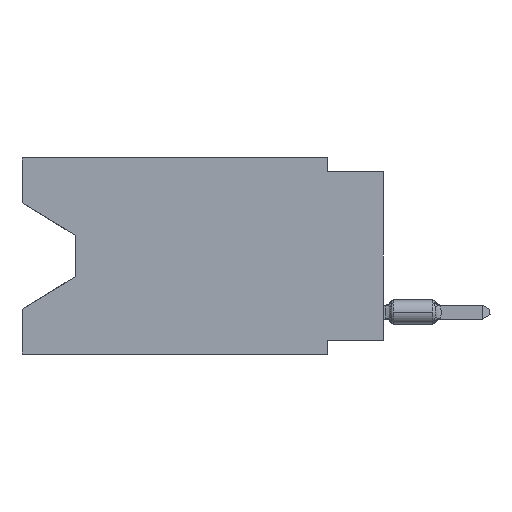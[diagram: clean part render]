
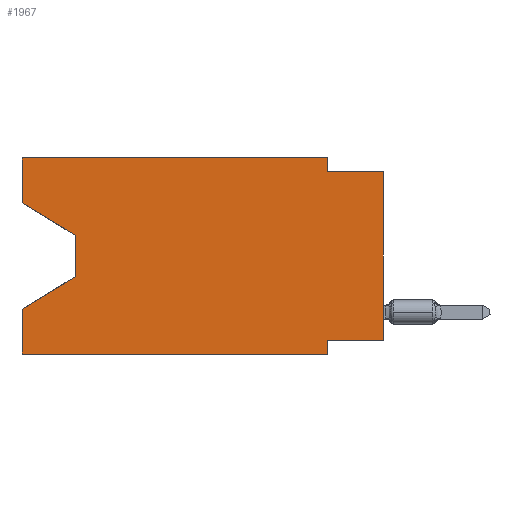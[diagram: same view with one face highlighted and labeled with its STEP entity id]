
A CAD part, left-side view. The second image highlights one B-rep face of the part: STEP entity #1967.
In plain terms, the highlighted planar face has unit normal (-1, 0, 0).
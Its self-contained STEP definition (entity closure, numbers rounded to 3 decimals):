
#152 = EDGE_CURVE ( 'NONE', #29118, #13031, #9220, .T. ) ;
#993 = CARTESIAN_POINT ( 'NONE',  ( 0., 16.383, -8.89 ) ) ;
#1120 = LINE ( 'NONE', #49168, #19352 ) ;
#1580 = CARTESIAN_POINT ( 'NONE',  ( 0., 0., -8.255 ) ) ;
#1967 = ADVANCED_FACE ( 'NONE', ( #51818 ), #21676, .F. ) ;
#2218 = DIRECTION ( 'NONE',  ( 0., -0.855, -0.519 ) ) ;
#2401 = LINE ( 'NONE', #15149, #39441 ) ;
#3089 = ORIENTED_EDGE ( 'NONE', *, *, #32509, .F. ) ;
#3797 = VECTOR ( 'NONE', #8239, 1000. ) ;
#4274 = EDGE_CURVE ( 'NONE', #53425, #5177, #39227, .T. ) ;
#4818 = CARTESIAN_POINT ( 'NONE',  ( 0., 16.383, -2.038 ) ) ;
#5027 = CARTESIAN_POINT ( 'NONE',  ( 0., 13.97, -3.505 ) ) ;
#5177 = VERTEX_POINT ( 'NONE', #44967 ) ;
#6761 = EDGE_CURVE ( 'NONE', #54355, #32090, #35703, .T. ) ;
#7062 = DIRECTION ( 'NONE',  ( 0., 1., 0. ) ) ;
#7073 = CARTESIAN_POINT ( 'NONE',  ( 0., 0., -8.255 ) ) ;
#8239 = DIRECTION ( 'NONE',  ( 0., 0., -1. ) ) ;
#8268 = VECTOR ( 'NONE', #56622, 1000. ) ;
#8330 = EDGE_CURVE ( 'NONE', #24706, #37891, #1120, .T. ) ;
#9220 = LINE ( 'NONE', #35254, #9801 ) ;
#9801 = VECTOR ( 'NONE', #54073, 1000. ) ;
#10299 = EDGE_CURVE ( 'NONE', #13031, #13612, #56295, .T. ) ;
#10389 = EDGE_CURVE ( 'NONE', #54650, #53425, #44946, .T. ) ;
#11003 = DIRECTION ( 'NONE',  ( 0., -1., 0. ) ) ;
#13031 = VERTEX_POINT ( 'NONE', #53365 ) ;
#13605 = ORIENTED_EDGE ( 'NONE', *, *, #25363, .T. ) ;
#13610 = CARTESIAN_POINT ( 'NONE',  ( 0., 2.54, -8.255 ) ) ;
#13612 = VERTEX_POINT ( 'NONE', #30114 ) ;
#15149 = CARTESIAN_POINT ( 'NONE',  ( 0., 16.383, 0. ) ) ;
#15272 = ORIENTED_EDGE ( 'NONE', *, *, #56501, .F. ) ;
#17179 = CARTESIAN_POINT ( 'NONE',  ( 0., 2.54, 0. ) ) ;
#19271 = CARTESIAN_POINT ( 'NONE',  ( 0., 16.383, -2.038 ) ) ;
#19352 = VECTOR ( 'NONE', #45099, 1000. ) ;
#19777 = VECTOR ( 'NONE', #30908, 1000. ) ;
#20022 = DIRECTION ( 'NONE',  ( 0., 0., 1. ) ) ;
#20681 = CARTESIAN_POINT ( 'NONE',  ( 0., 13.97, -5.385 ) ) ;
#21676 = PLANE ( 'NONE',  #21934 ) ;
#21934 = AXIS2_PLACEMENT_3D ( 'NONE', #56758, #43973, #48053 ) ;
#22174 = CARTESIAN_POINT ( 'NONE',  ( 0., 16.383, 0. ) ) ;
#23018 = LINE ( 'NONE', #19271, #24109 ) ;
#23809 = VECTOR ( 'NONE', #27017, 1000. ) ;
#23847 = ORIENTED_EDGE ( 'NONE', *, *, #6761, .T. ) ;
#24006 = VECTOR ( 'NONE', #7062, 1000. ) ;
#24109 = VECTOR ( 'NONE', #2218, 1000. ) ;
#24706 = VERTEX_POINT ( 'NONE', #7073 ) ;
#24864 = LINE ( 'NONE', #39329, #19777 ) ;
#25363 = EDGE_CURVE ( 'NONE', #53541, #54650, #23018, .T. ) ;
#25738 = ORIENTED_EDGE ( 'NONE', *, *, #8330, .T. ) ;
#27017 = DIRECTION ( 'NONE',  ( 0., -1., 0. ) ) ;
#29118 = VERTEX_POINT ( 'NONE', #22174 ) ;
#29225 = VERTEX_POINT ( 'NONE', #13610 ) ;
#29442 = EDGE_CURVE ( 'NONE', #13612, #37891, #36758, .T. ) ;
#30114 = CARTESIAN_POINT ( 'NONE',  ( 0., 2.54, -0.635 ) ) ;
#30908 = DIRECTION ( 'NONE',  ( 0., 0., -1. ) ) ;
#31626 = DIRECTION ( 'NONE',  ( 0., 0., -1. ) ) ;
#31807 = ORIENTED_EDGE ( 'NONE', *, *, #10389, .T. ) ;
#32090 = VERTEX_POINT ( 'NONE', #50246 ) ;
#32509 = EDGE_CURVE ( 'NONE', #53541, #29118, #2401, .T. ) ;
#34305 = VECTOR ( 'NONE', #31626, 1000. ) ;
#34629 = CARTESIAN_POINT ( 'NONE',  ( 0., 13.97, -3.505 ) ) ;
#34659 = ORIENTED_EDGE ( 'NONE', *, *, #50951, .F. ) ;
#35254 = CARTESIAN_POINT ( 'NONE',  ( 0., 16.383, 0. ) ) ;
#35598 = CARTESIAN_POINT ( 'NONE',  ( 0., 0., -0.635 ) ) ;
#35703 = LINE ( 'NONE', #993, #23809 ) ;
#36758 = LINE ( 'NONE', #37341, #54471 ) ;
#36892 = LINE ( 'NONE', #1580, #24006 ) ;
#37341 = CARTESIAN_POINT ( 'NONE',  ( 0., 0., -0.635 ) ) ;
#37442 = DIRECTION ( 'NONE',  ( 0., 0., 1. ) ) ;
#37891 = VERTEX_POINT ( 'NONE', #35598 ) ;
#39180 = EDGE_CURVE ( 'NONE', #29225, #32090, #24864, .T. ) ;
#39227 = LINE ( 'NONE', #20681, #8268 ) ;
#39329 = CARTESIAN_POINT ( 'NONE',  ( 0., 2.54, -8.89 ) ) ;
#39441 = VECTOR ( 'NONE', #20022, 1000. ) ;
#39917 = EDGE_LOOP ( 'NONE', ( #13605, #31807, #40950, #15272, #23847, #53342, #34659, #25738, #49713, #47643, #41933, #3089 ) ) ;
#40950 = ORIENTED_EDGE ( 'NONE', *, *, #4274, .T. ) ;
#41933 = ORIENTED_EDGE ( 'NONE', *, *, #152, .F. ) ;
#43973 = DIRECTION ( 'NONE',  ( 1., 0., 0. ) ) ;
#44946 = LINE ( 'NONE', #5027, #34305 ) ;
#44967 = CARTESIAN_POINT ( 'NONE',  ( 0., 16.383, -6.852 ) ) ;
#45099 = DIRECTION ( 'NONE',  ( 0., 0., 1. ) ) ;
#47643 = ORIENTED_EDGE ( 'NONE', *, *, #10299, .F. ) ;
#48053 = DIRECTION ( 'NONE',  ( 0., 0., -1. ) ) ;
#48243 = CARTESIAN_POINT ( 'NONE',  ( 0., 13.97, -5.385 ) ) ;
#49158 = VECTOR ( 'NONE', #37442, 1000. ) ;
#49168 = CARTESIAN_POINT ( 'NONE',  ( 0., 0., 0. ) ) ;
#49713 = ORIENTED_EDGE ( 'NONE', *, *, #29442, .F. ) ;
#50189 = CARTESIAN_POINT ( 'NONE',  ( 0., 16.383, 0. ) ) ;
#50246 = CARTESIAN_POINT ( 'NONE',  ( 0., 2.54, -8.89 ) ) ;
#50951 = EDGE_CURVE ( 'NONE', #24706, #29225, #36892, .T. ) ;
#51818 = FACE_OUTER_BOUND ( 'NONE', #39917, .T. ) ;
#53342 = ORIENTED_EDGE ( 'NONE', *, *, #39180, .F. ) ;
#53365 = CARTESIAN_POINT ( 'NONE',  ( 0., 2.54, 0. ) ) ;
#53425 = VERTEX_POINT ( 'NONE', #48243 ) ;
#53541 = VERTEX_POINT ( 'NONE', #4818 ) ;
#54073 = DIRECTION ( 'NONE',  ( 0., -1., 0. ) ) ;
#54237 = LINE ( 'NONE', #50189, #49158 ) ;
#54355 = VERTEX_POINT ( 'NONE', #55650 ) ;
#54471 = VECTOR ( 'NONE', #11003, 1000. ) ;
#54650 = VERTEX_POINT ( 'NONE', #34629 ) ;
#55650 = CARTESIAN_POINT ( 'NONE',  ( 0., 16.383, -8.89 ) ) ;
#56295 = LINE ( 'NONE', #17179, #3797 ) ;
#56501 = EDGE_CURVE ( 'NONE', #54355, #5177, #54237, .T. ) ;
#56622 = DIRECTION ( 'NONE',  ( 0., 0.855, -0.519 ) ) ;
#56758 = CARTESIAN_POINT ( 'NONE',  ( 0., 16.383, 0. ) ) ;
